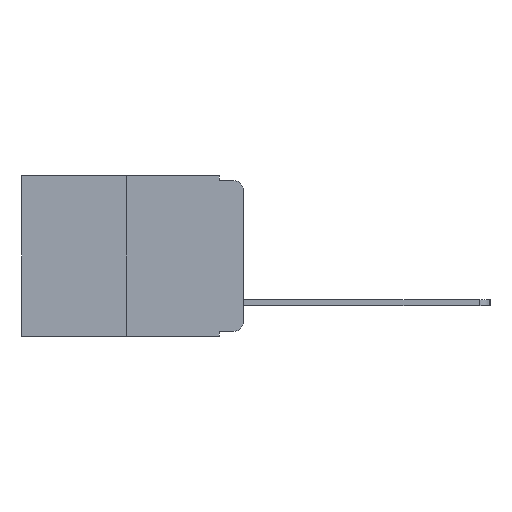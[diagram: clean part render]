
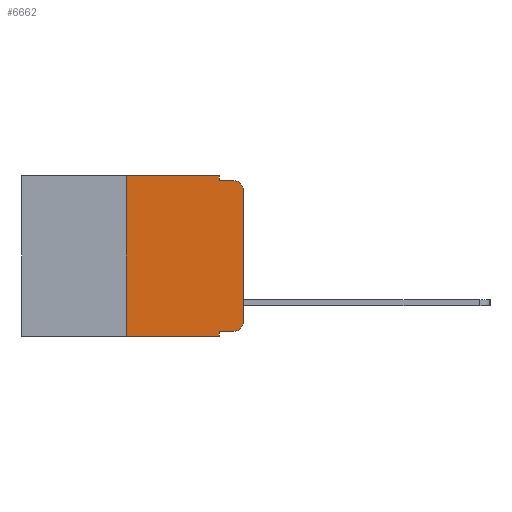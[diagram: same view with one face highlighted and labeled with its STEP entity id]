
A CAD part, left-side view. The second image highlights one B-rep face of the part: STEP entity #6662.
In plain terms, the highlighted planar face has unit normal (-1, 0, 0).
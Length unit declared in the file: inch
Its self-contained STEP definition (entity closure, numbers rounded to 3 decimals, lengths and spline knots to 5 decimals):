
#2 = CARTESIAN_POINT ( 'NONE',  ( 0., 0., -0.313 ) ) ;
#101 = ORIENTED_EDGE ( 'NONE', *, *, #9312, .T. ) ;
#274 = EDGE_CURVE ( 'NONE', #12814, #4769, #8397, .T. ) ;
#406 = VECTOR ( 'NONE', #7087, 39.37008 ) ;
#755 = VERTEX_POINT ( 'NONE', #12322 ) ;
#847 = DIRECTION ( 'NONE',  ( 0., 0., 1. ) ) ;
#932 = VERTEX_POINT ( 'NONE', #8106 ) ;
#1321 = CARTESIAN_POINT ( 'NONE',  ( 0., 0.02, -0.01 ) ) ;
#1377 = VECTOR ( 'NONE', #847, 39.37008 ) ;
#1502 = VECTOR ( 'NONE', #5241, 39.37008 ) ;
#1714 = PLANE ( 'NONE',  #6508 ) ;
#1760 = CARTESIAN_POINT ( 'NONE',  ( 0., 0.473, 0. ) ) ;
#1833 = LINE ( 'NONE', #7553, #1377 ) ;
#2219 = VERTEX_POINT ( 'NONE', #13101 ) ;
#3011 = VERTEX_POINT ( 'NONE', #12812 ) ;
#3113 = DIRECTION ( 'NONE',  ( 1., 0., 0. ) ) ;
#3315 = ORIENTED_EDGE ( 'NONE', *, *, #12116, .F. ) ;
#3685 = ORIENTED_EDGE ( 'NONE', *, *, #6852, .T. ) ;
#4153 = VECTOR ( 'NONE', #14713, 39.37008 ) ;
#4165 = CARTESIAN_POINT ( 'NONE',  ( 0., 0.051, 0. ) ) ;
#4255 = CARTESIAN_POINT ( 'NONE',  ( 0., 0.25, 0. ) ) ;
#4427 = ORIENTED_EDGE ( 'NONE', *, *, #11409, .F. ) ;
#4536 = ORIENTED_EDGE ( 'NONE', *, *, #274, .T. ) ;
#4585 = ORIENTED_EDGE ( 'NONE', *, *, #14789, .T. ) ;
#4648 = ORIENTED_EDGE ( 'NONE', *, *, #14148, .F. ) ;
#4668 = FACE_OUTER_BOUND ( 'NONE', #5944, .T. ) ;
#4671 = CARTESIAN_POINT ( 'NONE',  ( 0., 0.051, -0.343 ) ) ;
#4681 = ORIENTED_EDGE ( 'NONE', *, *, #10725, .T. ) ;
#4720 = VECTOR ( 'NONE', #5177, 39.37008 ) ;
#4769 = VERTEX_POINT ( 'NONE', #13167 ) ;
#4809 = ORIENTED_EDGE ( 'NONE', *, *, #13482, .F. ) ;
#4901 = ORIENTED_EDGE ( 'NONE', *, *, #6044, .F. ) ;
#5177 = DIRECTION ( 'NONE',  ( 0., -1., 0. ) ) ;
#5241 = DIRECTION ( 'NONE',  ( 0., -1., 0. ) ) ;
#5458 = DIRECTION ( 'NONE',  ( 0., 0., -1. ) ) ;
#5489 = LINE ( 'NONE', #12055, #1502 ) ;
#5647 = DIRECTION ( 'NONE',  ( -1., 0., 0. ) ) ;
#5678 = CARTESIAN_POINT ( 'NONE',  ( 0., 0.473, 0. ) ) ;
#5944 = EDGE_LOOP ( 'NONE', ( #4536, #4585, #4648, #4809, #4901, #3315, #3685, #4427, #4681, #101 ) ) ;
#5948 = VERTEX_POINT ( 'NONE', #11138 ) ;
#6044 = EDGE_CURVE ( 'NONE', #6618, #755, #10140, .T. ) ;
#6508 = AXIS2_PLACEMENT_3D ( 'NONE', #5678, #3113, #11369 ) ;
#6618 = VERTEX_POINT ( 'NONE', #4255 ) ;
#6620 = LINE ( 'NONE', #13678, #9324 ) ;
#6662 = ADVANCED_FACE ( 'NONE', ( #4668 ), #1714, .F. ) ;
#6852 = EDGE_CURVE ( 'NONE', #2219, #13317, #5489, .T. ) ;
#6921 = VERTEX_POINT ( 'NONE', #1321 ) ;
#6976 = CARTESIAN_POINT ( 'NONE',  ( 0., 0.02, -0.313 ) ) ;
#7087 = DIRECTION ( 'NONE',  ( 0., -1., 0. ) ) ;
#7358 = DIRECTION ( 'NONE',  ( 0., -1., 0. ) ) ;
#7428 = CARTESIAN_POINT ( 'NONE',  ( 0., 0.051, 0. ) ) ;
#7553 = CARTESIAN_POINT ( 'NONE',  ( 0., 0.25, 0. ) ) ;
#8106 = CARTESIAN_POINT ( 'NONE',  ( 0., 0.051, -0.333 ) ) ;
#8191 = DIRECTION ( 'NONE',  ( 0., 0., -1. ) ) ;
#8397 = LINE ( 'NONE', #14663, #13574 ) ;
#9161 = VECTOR ( 'NONE', #5458, 39.37008 ) ;
#9312 = EDGE_CURVE ( 'NONE', #3011, #12814, #10990, .T. ) ;
#9324 = VECTOR ( 'NONE', #7358, 39.37008 ) ;
#10140 = LINE ( 'NONE', #1760, #406 ) ;
#10446 = LINE ( 'NONE', #7428, #4153 ) ;
#10725 = EDGE_CURVE ( 'NONE', #932, #3011, #6620, .T. ) ;
#10952 = CARTESIAN_POINT ( 'NONE',  ( 0., 0.051, -0.01 ) ) ;
#10990 = CIRCLE ( 'NONE', #13271, 0.02 ) ;
#11138 = CARTESIAN_POINT ( 'NONE',  ( 0., 0.051, -0.01 ) ) ;
#11369 = DIRECTION ( 'NONE',  ( 0., 0., -1. ) ) ;
#11409 = EDGE_CURVE ( 'NONE', #932, #13317, #14305, .T. ) ;
#12055 = CARTESIAN_POINT ( 'NONE',  ( 0., 0.473, -0.343 ) ) ;
#12116 = EDGE_CURVE ( 'NONE', #2219, #6618, #1833, .T. ) ;
#12184 = DIRECTION ( 'NONE',  ( 0., 0., 1. ) ) ;
#12322 = CARTESIAN_POINT ( 'NONE',  ( 0., 0.051, 0. ) ) ;
#12350 = CARTESIAN_POINT ( 'NONE',  ( 0., 0.02, -0.03 ) ) ;
#12812 = CARTESIAN_POINT ( 'NONE',  ( 0., 0.02, -0.333 ) ) ;
#12814 = VERTEX_POINT ( 'NONE', #2 ) ;
#13101 = CARTESIAN_POINT ( 'NONE',  ( 0., 0.25, -0.343 ) ) ;
#13167 = CARTESIAN_POINT ( 'NONE',  ( 0., 0., -0.03 ) ) ;
#13271 = AXIS2_PLACEMENT_3D ( 'NONE', #6976, #14371, #8191 ) ;
#13317 = VERTEX_POINT ( 'NONE', #4671 ) ;
#13370 = DIRECTION ( 'NONE',  ( 0., 0., -1. ) ) ;
#13482 = EDGE_CURVE ( 'NONE', #755, #5948, #10446, .T. ) ;
#13574 = VECTOR ( 'NONE', #12184, 39.37008 ) ;
#13678 = CARTESIAN_POINT ( 'NONE',  ( 0., 0.051, -0.333 ) ) ;
#13971 = LINE ( 'NONE', #10952, #4720 ) ;
#14124 = CIRCLE ( 'NONE', #15026, 0.02 ) ;
#14148 = EDGE_CURVE ( 'NONE', #5948, #6921, #13971, .T. ) ;
#14305 = LINE ( 'NONE', #4165, #9161 ) ;
#14371 = DIRECTION ( 'NONE',  ( -1., 0., 0. ) ) ;
#14663 = CARTESIAN_POINT ( 'NONE',  ( 0., 0., 0. ) ) ;
#14713 = DIRECTION ( 'NONE',  ( 0., 0., -1. ) ) ;
#14789 = EDGE_CURVE ( 'NONE', #4769, #6921, #14124, .T. ) ;
#15026 = AXIS2_PLACEMENT_3D ( 'NONE', #12350, #5647, #13370 ) ;
